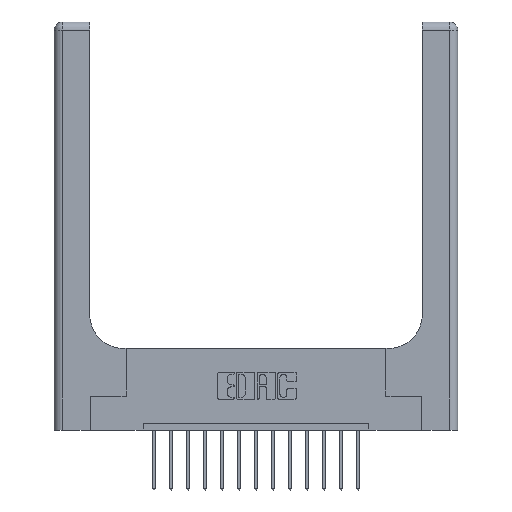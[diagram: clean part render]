
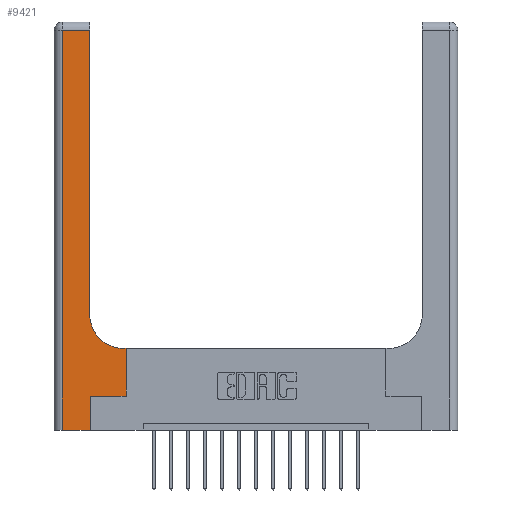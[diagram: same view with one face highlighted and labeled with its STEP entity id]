
A CAD part, top view. The second image highlights one B-rep face of the part: STEP entity #9421.
In plain terms, the highlighted planar face has unit normal (0, 0, 1).
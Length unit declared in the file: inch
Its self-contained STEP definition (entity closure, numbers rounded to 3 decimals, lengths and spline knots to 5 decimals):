
#65 = DIRECTION ( 'NONE',  ( 0., 0., -1. ) ) ;
#350 = ORIENTED_EDGE ( 'NONE', *, *, #17563, .T. ) ;
#416 = ORIENTED_EDGE ( 'NONE', *, *, #10914, .T. ) ;
#781 = DIRECTION ( 'NONE',  ( 0., 0., -1. ) ) ;
#938 = EDGE_CURVE ( 'NONE', #6850, #12309, #13567, .T. ) ;
#1215 = VECTOR ( 'NONE', #10626, 39.37008 ) ;
#1659 = CARTESIAN_POINT ( 'NONE',  ( 0.26, 0.6, 0.37 ) ) ;
#2014 = CARTESIAN_POINT ( 'NONE',  ( 0.51, 0.6, 0.37 ) ) ;
#2121 = PLANE ( 'NONE',  #2357 ) ;
#2357 = AXIS2_PLACEMENT_3D ( 'NONE', #8903, #781, #7627 ) ;
#2491 = CARTESIAN_POINT ( 'NONE',  ( 0.51, 0.85, 0.37 ) ) ;
#3512 = VECTOR ( 'NONE', #17108, 39.37008 ) ;
#3592 = CARTESIAN_POINT ( 'NONE',  ( 0., 0., 0.37 ) ) ;
#3625 = ORIENTED_EDGE ( 'NONE', *, *, #3726, .T. ) ;
#3663 = LINE ( 'NONE', #6825, #8527 ) ;
#3726 = EDGE_CURVE ( 'NONE', #11908, #6850, #11348, .T. ) ;
#4055 = VECTOR ( 'NONE', #13878, 39.37008 ) ;
#4143 = CARTESIAN_POINT ( 'NONE',  ( 0., 2.94, 0.37 ) ) ;
#4660 = CARTESIAN_POINT ( 'NONE',  ( 0.26, 2.94, 0.37 ) ) ;
#5158 = VECTOR ( 'NONE', #9319, 39.37008 ) ;
#5516 = DIRECTION ( 'NONE',  ( 1., 0., 0. ) ) ;
#5846 = VERTEX_POINT ( 'NONE', #9315 ) ;
#5868 = LINE ( 'NONE', #9803, #4055 ) ;
#6691 = EDGE_CURVE ( 'NONE', #7174, #13691, #3663, .T. ) ;
#6796 = DIRECTION ( 'NONE',  ( 0., 1., 0. ) ) ;
#6825 = CARTESIAN_POINT ( 'NONE',  ( 0.528, 0.25, 0.37 ) ) ;
#6850 = VERTEX_POINT ( 'NONE', #11732 ) ;
#6918 = LINE ( 'NONE', #1659, #10676 ) ;
#7174 = VERTEX_POINT ( 'NONE', #8957 ) ;
#7627 = DIRECTION ( 'NONE',  ( -1., 0., 0. ) ) ;
#8245 = VERTEX_POINT ( 'NONE', #11647 ) ;
#8527 = VECTOR ( 'NONE', #12280, 39.37008 ) ;
#8661 = CARTESIAN_POINT ( 'NONE',  ( 0.528, 0.6, 0.37 ) ) ;
#8873 = VECTOR ( 'NONE', #15907, 39.37008 ) ;
#8903 = CARTESIAN_POINT ( 'NONE',  ( 0., 3., 0.37 ) ) ;
#8957 = CARTESIAN_POINT ( 'NONE',  ( 0.528, 0.25, 0.37 ) ) ;
#9239 = EDGE_CURVE ( 'NONE', #8245, #17244, #5868, .T. ) ;
#9315 = CARTESIAN_POINT ( 'NONE',  ( 0.06, 2.94, 0.37 ) ) ;
#9319 = DIRECTION ( 'NONE',  ( -1., 0., 0. ) ) ;
#9358 = AXIS2_PLACEMENT_3D ( 'NONE', #2491, #65, #5516 ) ;
#9421 = ADVANCED_FACE ( 'NONE', ( #15647 ), #2121, .F. ) ;
#9803 = CARTESIAN_POINT ( 'NONE',  ( 0.265, 0., 0.37 ) ) ;
#10162 = EDGE_CURVE ( 'NONE', #12112, #8245, #11705, .T. ) ;
#10351 = ORIENTED_EDGE ( 'NONE', *, *, #9239, .T. ) ;
#10626 = DIRECTION ( 'NONE',  ( 1., 0., 0. ) ) ;
#10676 = VECTOR ( 'NONE', #11210, 39.37008 ) ;
#10914 = EDGE_CURVE ( 'NONE', #13691, #11908, #6918, .T. ) ;
#11210 = DIRECTION ( 'NONE',  ( -1., 0., 0. ) ) ;
#11348 = CIRCLE ( 'NONE', #9358, 0.25 ) ;
#11402 = LINE ( 'NONE', #13075, #8873 ) ;
#11647 = CARTESIAN_POINT ( 'NONE',  ( 0.265, 0., 0.37 ) ) ;
#11705 = LINE ( 'NONE', #3592, #3512 ) ;
#11732 = CARTESIAN_POINT ( 'NONE',  ( 0.26, 0.85, 0.37 ) ) ;
#11908 = VERTEX_POINT ( 'NONE', #2014 ) ;
#11940 = EDGE_CURVE ( 'NONE', #12309, #5846, #16330, .T. ) ;
#12112 = VERTEX_POINT ( 'NONE', #15005 ) ;
#12280 = DIRECTION ( 'NONE',  ( 0., 1., 0. ) ) ;
#12309 = VERTEX_POINT ( 'NONE', #4660 ) ;
#12541 = ORIENTED_EDGE ( 'NONE', *, *, #10162, .T. ) ;
#12550 = ORIENTED_EDGE ( 'NONE', *, *, #938, .T. ) ;
#13049 = EDGE_CURVE ( 'NONE', #5846, #12112, #11402, .T. ) ;
#13075 = CARTESIAN_POINT ( 'NONE',  ( 0.06, 3., 0.37 ) ) ;
#13284 = ORIENTED_EDGE ( 'NONE', *, *, #6691, .T. ) ;
#13368 = LINE ( 'NONE', #17367, #1215 ) ;
#13567 = LINE ( 'NONE', #13834, #14078 ) ;
#13651 = EDGE_LOOP ( 'NONE', ( #12550, #16082, #15224, #12541, #10351, #350, #13284, #416, #3625 ) ) ;
#13691 = VERTEX_POINT ( 'NONE', #8661 ) ;
#13834 = CARTESIAN_POINT ( 'NONE',  ( 0.26, 3., 0.37 ) ) ;
#13878 = DIRECTION ( 'NONE',  ( 0., 1., 0. ) ) ;
#14078 = VECTOR ( 'NONE', #6796, 39.37008 ) ;
#15005 = CARTESIAN_POINT ( 'NONE',  ( 0.06, 0., 0.37 ) ) ;
#15224 = ORIENTED_EDGE ( 'NONE', *, *, #13049, .T. ) ;
#15250 = CARTESIAN_POINT ( 'NONE',  ( 0.265, 0.25, 0.37 ) ) ;
#15647 = FACE_OUTER_BOUND ( 'NONE', #13651, .T. ) ;
#15907 = DIRECTION ( 'NONE',  ( 0., -1., 0. ) ) ;
#16082 = ORIENTED_EDGE ( 'NONE', *, *, #11940, .T. ) ;
#16330 = LINE ( 'NONE', #4143, #5158 ) ;
#17108 = DIRECTION ( 'NONE',  ( 1., 0., 0. ) ) ;
#17244 = VERTEX_POINT ( 'NONE', #15250 ) ;
#17367 = CARTESIAN_POINT ( 'NONE',  ( 0.265, 0.25, 0.37 ) ) ;
#17563 = EDGE_CURVE ( 'NONE', #17244, #7174, #13368, .T. ) ;
